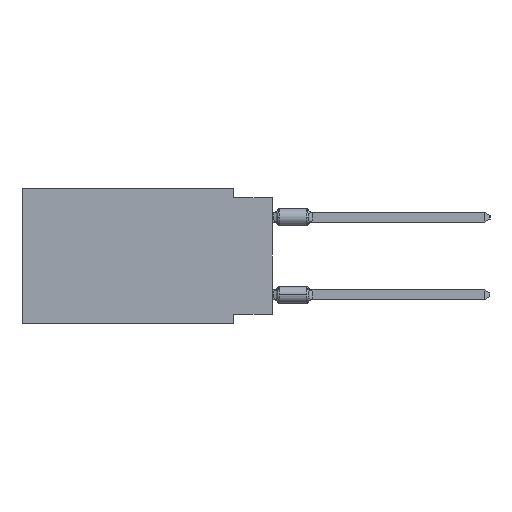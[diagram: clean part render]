
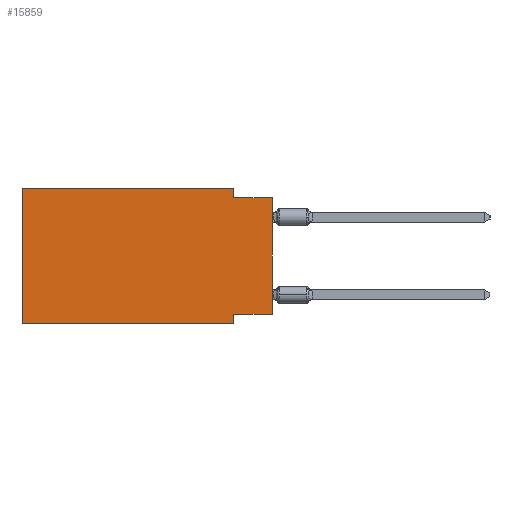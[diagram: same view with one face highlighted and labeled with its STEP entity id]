
A CAD part, left-side view. The second image highlights one B-rep face of the part: STEP entity #15859.
In plain terms, the highlighted planar face has unit normal (-1, 0, 0).
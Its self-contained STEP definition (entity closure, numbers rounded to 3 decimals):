
#534 = PLANE ( 'NONE',  #27855 ) ;
#819 = CARTESIAN_POINT ( 'NONE',  ( 0., 2.54, -8.89 ) ) ;
#1313 = LINE ( 'NONE', #1781, #19749 ) ;
#1781 = CARTESIAN_POINT ( 'NONE',  ( 0., 0., -8.255 ) ) ;
#1862 = CARTESIAN_POINT ( 'NONE',  ( 0., 0., 0. ) ) ;
#1893 = ORIENTED_EDGE ( 'NONE', *, *, #38630, .T. ) ;
#2470 = VERTEX_POINT ( 'NONE', #10339 ) ;
#3276 = CARTESIAN_POINT ( 'NONE',  ( 0., 2.54, -8.255 ) ) ;
#3430 = CARTESIAN_POINT ( 'NONE',  ( 0., 2.54, 0. ) ) ;
#3880 = DIRECTION ( 'NONE',  ( 0., -1., 0. ) ) ;
#5384 = VECTOR ( 'NONE', #8294, 1000. ) ;
#7213 = CARTESIAN_POINT ( 'NONE',  ( 0., 16.383, -8.89 ) ) ;
#8294 = DIRECTION ( 'NONE',  ( 0., 0., 1. ) ) ;
#8653 = DIRECTION ( 'NONE',  ( 0., -1., 0. ) ) ;
#8811 = DIRECTION ( 'NONE',  ( 0., 0., -1. ) ) ;
#9472 = VERTEX_POINT ( 'NONE', #819 ) ;
#9737 = VERTEX_POINT ( 'NONE', #25636 ) ;
#10339 = CARTESIAN_POINT ( 'NONE',  ( 0., 2.54, -0.635 ) ) ;
#10759 = ORIENTED_EDGE ( 'NONE', *, *, #33070, .F. ) ;
#11160 = ORIENTED_EDGE ( 'NONE', *, *, #36989, .F. ) ;
#11605 = CARTESIAN_POINT ( 'NONE',  ( 0., 16.383, 0. ) ) ;
#12312 = ORIENTED_EDGE ( 'NONE', *, *, #38660, .F. ) ;
#12352 = CARTESIAN_POINT ( 'NONE',  ( 0., 2.54, -8.89 ) ) ;
#15612 = DIRECTION ( 'NONE',  ( 0., 0., 1. ) ) ;
#15859 = ADVANCED_FACE ( 'NONE', ( #32969 ), #534, .F. ) ;
#16225 = DIRECTION ( 'NONE',  ( 0., 1., 0. ) ) ;
#16335 = LINE ( 'NONE', #30780, #34114 ) ;
#16507 = EDGE_CURVE ( 'NONE', #44048, #9737, #41170, .T. ) ;
#16808 = DIRECTION ( 'NONE',  ( 0., 0., -1. ) ) ;
#16929 = ORIENTED_EDGE ( 'NONE', *, *, #36776, .F. ) ;
#19749 = VECTOR ( 'NONE', #16225, 1000. ) ;
#20210 = VECTOR ( 'NONE', #15612, 1000. ) ;
#20489 = CARTESIAN_POINT ( 'NONE',  ( 0., 0., -8.255 ) ) ;
#20618 = LINE ( 'NONE', #31515, #28201 ) ;
#21182 = VERTEX_POINT ( 'NONE', #7213 ) ;
#22343 = LINE ( 'NONE', #36565, #32589 ) ;
#22505 = LINE ( 'NONE', #11605, #5384 ) ;
#23983 = VERTEX_POINT ( 'NONE', #3430 ) ;
#25636 = CARTESIAN_POINT ( 'NONE',  ( 0., 0., -0.635 ) ) ;
#25789 = VECTOR ( 'NONE', #8653, 1000. ) ;
#25794 = ORIENTED_EDGE ( 'NONE', *, *, #40856, .F. ) ;
#26558 = DIRECTION ( 'NONE',  ( 0., 0., -1. ) ) ;
#27855 = AXIS2_PLACEMENT_3D ( 'NONE', #29419, #37220, #26558 ) ;
#28201 = VECTOR ( 'NONE', #45938, 1000. ) ;
#29419 = CARTESIAN_POINT ( 'NONE',  ( 0., 16.383, 0. ) ) ;
#30780 = CARTESIAN_POINT ( 'NONE',  ( 0., 2.54, 0. ) ) ;
#31515 = CARTESIAN_POINT ( 'NONE',  ( 0., 16.383, 0. ) ) ;
#32589 = VECTOR ( 'NONE', #3880, 1000. ) ;
#32969 = FACE_OUTER_BOUND ( 'NONE', #44472, .T. ) ;
#33070 = EDGE_CURVE ( 'NONE', #46114, #9472, #41243, .T. ) ;
#34114 = VECTOR ( 'NONE', #16808, 1000. ) ;
#36565 = CARTESIAN_POINT ( 'NONE',  ( 0., 0., -0.635 ) ) ;
#36776 = EDGE_CURVE ( 'NONE', #21182, #45570, #22505, .T. ) ;
#36841 = ORIENTED_EDGE ( 'NONE', *, *, #16507, .T. ) ;
#36989 = EDGE_CURVE ( 'NONE', #23983, #2470, #16335, .T. ) ;
#37220 = DIRECTION ( 'NONE',  ( 1., 0., 0. ) ) ;
#37780 = LINE ( 'NONE', #42027, #25789 ) ;
#38232 = VECTOR ( 'NONE', #8811, 1000. ) ;
#38630 = EDGE_CURVE ( 'NONE', #21182, #9472, #37780, .T. ) ;
#38660 = EDGE_CURVE ( 'NONE', #44048, #46114, #1313, .T. ) ;
#38859 = EDGE_CURVE ( 'NONE', #2470, #9737, #22343, .T. ) ;
#39746 = ORIENTED_EDGE ( 'NONE', *, *, #38859, .F. ) ;
#40807 = CARTESIAN_POINT ( 'NONE',  ( 0., 16.383, 0. ) ) ;
#40856 = EDGE_CURVE ( 'NONE', #45570, #23983, #20618, .T. ) ;
#41170 = LINE ( 'NONE', #1862, #20210 ) ;
#41243 = LINE ( 'NONE', #12352, #38232 ) ;
#42027 = CARTESIAN_POINT ( 'NONE',  ( 0., 16.383, -8.89 ) ) ;
#44048 = VERTEX_POINT ( 'NONE', #20489 ) ;
#44472 = EDGE_LOOP ( 'NONE', ( #36841, #39746, #11160, #25794, #16929, #1893, #10759, #12312 ) ) ;
#45570 = VERTEX_POINT ( 'NONE', #40807 ) ;
#45938 = DIRECTION ( 'NONE',  ( 0., -1., 0. ) ) ;
#46114 = VERTEX_POINT ( 'NONE', #3276 ) ;
